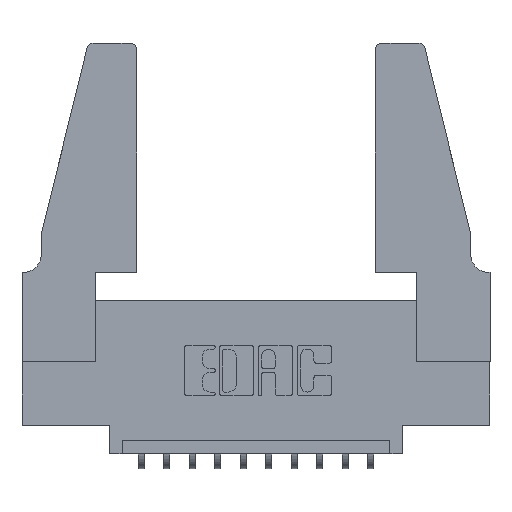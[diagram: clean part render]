
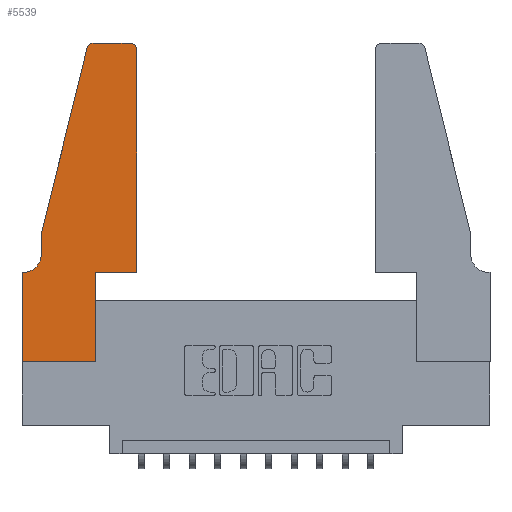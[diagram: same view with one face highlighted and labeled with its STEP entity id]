
A CAD part, top view. The second image highlights one B-rep face of the part: STEP entity #5539.
In plain terms, the highlighted planar face has unit normal (0, 0, 1).
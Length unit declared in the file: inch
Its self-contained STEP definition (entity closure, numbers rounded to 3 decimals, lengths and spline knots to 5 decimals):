
#28 = LINE ( 'NONE', #13842, #6927 ) ;
#29 = VECTOR ( 'NONE', #12628, 39.37008 ) ;
#161 = CARTESIAN_POINT ( 'NONE',  ( 0.25487, 1.22718, 0.37 ) ) ;
#336 = CARTESIAN_POINT ( 'NONE',  ( 0., 0.35, 0.37 ) ) ;
#365 = DIRECTION ( 'NONE',  ( 0., 0., 1. ) ) ;
#396 = CARTESIAN_POINT ( 'NONE',  ( 0.284, 1.25, 0.37 ) ) ;
#745 = VECTOR ( 'NONE', #5451, 39.37008 ) ;
#904 = EDGE_CURVE ( 'NONE', #2541, #1559, #2519, .T. ) ;
#1298 = DIRECTION ( 'NONE',  ( 0., 1., 0. ) ) ;
#1559 = VERTEX_POINT ( 'NONE', #4069 ) ;
#1693 = AXIS2_PLACEMENT_3D ( 'NONE', #8926, #6748, #2384 ) ;
#2105 = VERTEX_POINT ( 'NONE', #11267 ) ;
#2175 = EDGE_CURVE ( 'NONE', #1559, #9180, #10941, .T. ) ;
#2384 = DIRECTION ( 'NONE',  ( -1., 0., 0. ) ) ;
#2443 = LINE ( 'NONE', #10088, #3154 ) ;
#2477 = DIRECTION ( 'NONE',  ( 0., 1., 0. ) ) ;
#2519 = CIRCLE ( 'NONE', #9201, 0.03 ) ;
#2541 = VERTEX_POINT ( 'NONE', #13752 ) ;
#2682 = CARTESIAN_POINT ( 'NONE',  ( 0.0755, 0.5, 0.37 ) ) ;
#2744 = EDGE_CURVE ( 'NONE', #7398, #2541, #7820, .T. ) ;
#2819 = VERTEX_POINT ( 'NONE', #161 ) ;
#3118 = DIRECTION ( 'NONE',  ( 0., 0., 1. ) ) ;
#3154 = VECTOR ( 'NONE', #2477, 39.37008 ) ;
#3212 = ORIENTED_EDGE ( 'NONE', *, *, #13450, .T. ) ;
#3365 = EDGE_CURVE ( 'NONE', #11986, #6659, #7637, .T. ) ;
#3370 = AXIS2_PLACEMENT_3D ( 'NONE', #336, #3869, #9328 ) ;
#3598 = VECTOR ( 'NONE', #7036, 39.37008 ) ;
#3607 = EDGE_CURVE ( 'NONE', #14097, #11986, #5263, .T. ) ;
#3843 = CARTESIAN_POINT ( 'NONE',  ( 0., 0., 0.37 ) ) ;
#3869 = DIRECTION ( 'NONE',  ( 0., 0., 1. ) ) ;
#3981 = FACE_OUTER_BOUND ( 'NONE', #4562, .T. ) ;
#4015 = ORIENTED_EDGE ( 'NONE', *, *, #904, .T. ) ;
#4069 = CARTESIAN_POINT ( 'NONE',  ( 0.4205, 1.25, 0.37 ) ) ;
#4224 = CARTESIAN_POINT ( 'NONE',  ( 0.284, 1.22, 0.37 ) ) ;
#4493 = EDGE_CURVE ( 'NONE', #9180, #2819, #5408, .T. ) ;
#4562 = EDGE_LOOP ( 'NONE', ( #12270, #12605, #13029, #10360, #9900, #3212, #8169, #9021, #10271, #14172, #5743, #4015 ) ) ;
#4669 = DIRECTION ( 'NONE',  ( -1., 0., 0. ) ) ;
#4884 = CARTESIAN_POINT ( 'NONE',  ( 0., 0., 0.37 ) ) ;
#5263 = LINE ( 'NONE', #14032, #745 ) ;
#5343 = EDGE_CURVE ( 'NONE', #2105, #6304, #6221, .T. ) ;
#5358 = EDGE_CURVE ( 'NONE', #9306, #2105, #10856, .T. ) ;
#5408 = CIRCLE ( 'NONE', #13093, 0.03 ) ;
#5451 = DIRECTION ( 'NONE',  ( 0., -1., 0. ) ) ;
#5539 = ADVANCED_FACE ( 'NONE', ( #3981 ), #6946, .T. ) ;
#5743 = ORIENTED_EDGE ( 'NONE', *, *, #2744, .T. ) ;
#6221 = CIRCLE ( 'NONE', #1693, 0.07 ) ;
#6291 = CARTESIAN_POINT ( 'NONE',  ( 0.2865, 0.35, 0.37 ) ) ;
#6304 = VERTEX_POINT ( 'NONE', #11362 ) ;
#6640 = VECTOR ( 'NONE', #1298, 39.37008 ) ;
#6659 = VERTEX_POINT ( 'NONE', #8403 ) ;
#6748 = DIRECTION ( 'NONE',  ( 0., 0., -1. ) ) ;
#6750 = CARTESIAN_POINT ( 'NONE',  ( 0.4205, 1.22, 0.37 ) ) ;
#6927 = VECTOR ( 'NONE', #13789, 39.37008 ) ;
#6946 = PLANE ( 'NONE',  #3370 ) ;
#7036 = DIRECTION ( 'NONE',  ( 1., 0., 0. ) ) ;
#7398 = VERTEX_POINT ( 'NONE', #8034 ) ;
#7479 = EDGE_CURVE ( 'NONE', #2819, #9306, #11731, .T. ) ;
#7637 = LINE ( 'NONE', #3843, #11923 ) ;
#7773 = CARTESIAN_POINT ( 'NONE',  ( 0.4505, 0.35, 0.37 ) ) ;
#7820 = LINE ( 'NONE', #7773, #6640 ) ;
#8034 = CARTESIAN_POINT ( 'NONE',  ( 0.4505, 0.35, 0.37 ) ) ;
#8169 = ORIENTED_EDGE ( 'NONE', *, *, #3607, .T. ) ;
#8403 = CARTESIAN_POINT ( 'NONE',  ( 0.2865, 0., 0.37 ) ) ;
#8926 = CARTESIAN_POINT ( 'NONE',  ( 0.0055, 0.42, 0.37 ) ) ;
#8983 = EDGE_CURVE ( 'NONE', #11793, #7398, #12499, .T. ) ;
#9021 = ORIENTED_EDGE ( 'NONE', *, *, #3365, .T. ) ;
#9180 = VERTEX_POINT ( 'NONE', #396 ) ;
#9201 = AXIS2_PLACEMENT_3D ( 'NONE', #6750, #365, #10997 ) ;
#9306 = VERTEX_POINT ( 'NONE', #10143 ) ;
#9328 = DIRECTION ( 'NONE',  ( 1., 0., 0. ) ) ;
#9635 = CARTESIAN_POINT ( 'NONE',  ( 0.4505, 0.35, 0.37 ) ) ;
#9900 = ORIENTED_EDGE ( 'NONE', *, *, #5343, .T. ) ;
#10071 = CARTESIAN_POINT ( 'NONE',  ( 0.2605, 1.25, 0.37 ) ) ;
#10088 = CARTESIAN_POINT ( 'NONE',  ( 0.2865, 0.35, 0.37 ) ) ;
#10143 = CARTESIAN_POINT ( 'NONE',  ( 0.0755, 0.5, 0.37 ) ) ;
#10271 = ORIENTED_EDGE ( 'NONE', *, *, #12947, .T. ) ;
#10317 = VECTOR ( 'NONE', #12994, 39.37008 ) ;
#10360 = ORIENTED_EDGE ( 'NONE', *, *, #5358, .T. ) ;
#10856 = LINE ( 'NONE', #11466, #10317 ) ;
#10941 = LINE ( 'NONE', #10071, #11611 ) ;
#10997 = DIRECTION ( 'NONE',  ( 1., 0., 0. ) ) ;
#11267 = CARTESIAN_POINT ( 'NONE',  ( 0.0755, 0.42, 0.37 ) ) ;
#11362 = CARTESIAN_POINT ( 'NONE',  ( 0.0055, 0.35, 0.37 ) ) ;
#11425 = DIRECTION ( 'NONE',  ( 1., 0., 0. ) ) ;
#11466 = CARTESIAN_POINT ( 'NONE',  ( 0.0755, 0.5, 0.37 ) ) ;
#11611 = VECTOR ( 'NONE', #4669, 39.37008 ) ;
#11731 = LINE ( 'NONE', #2682, #29 ) ;
#11793 = VERTEX_POINT ( 'NONE', #6291 ) ;
#11877 = CARTESIAN_POINT ( 'NONE',  ( 0., 0.35, 0.37 ) ) ;
#11923 = VECTOR ( 'NONE', #12034, 39.37008 ) ;
#11986 = VERTEX_POINT ( 'NONE', #4884 ) ;
#12034 = DIRECTION ( 'NONE',  ( 1., 0., 0. ) ) ;
#12270 = ORIENTED_EDGE ( 'NONE', *, *, #2175, .T. ) ;
#12499 = LINE ( 'NONE', #9635, #3598 ) ;
#12605 = ORIENTED_EDGE ( 'NONE', *, *, #4493, .T. ) ;
#12628 = DIRECTION ( 'NONE',  ( -0.239, -0.971, 0. ) ) ;
#12947 = EDGE_CURVE ( 'NONE', #6659, #11793, #2443, .T. ) ;
#12994 = DIRECTION ( 'NONE',  ( 0., -1., 0. ) ) ;
#13029 = ORIENTED_EDGE ( 'NONE', *, *, #7479, .T. ) ;
#13093 = AXIS2_PLACEMENT_3D ( 'NONE', #4224, #3118, #11425 ) ;
#13450 = EDGE_CURVE ( 'NONE', #6304, #14097, #28, .T. ) ;
#13752 = CARTESIAN_POINT ( 'NONE',  ( 0.4505, 1.22, 0.37 ) ) ;
#13789 = DIRECTION ( 'NONE',  ( -1., 0., 0. ) ) ;
#13842 = CARTESIAN_POINT ( 'NONE',  ( 0.0755, 0.35, 0.37 ) ) ;
#14032 = CARTESIAN_POINT ( 'NONE',  ( 0., 0., 0.37 ) ) ;
#14097 = VERTEX_POINT ( 'NONE', #11877 ) ;
#14172 = ORIENTED_EDGE ( 'NONE', *, *, #8983, .T. ) ;
